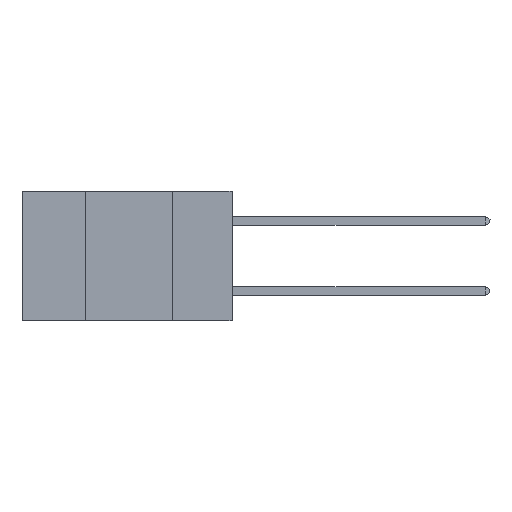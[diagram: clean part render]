
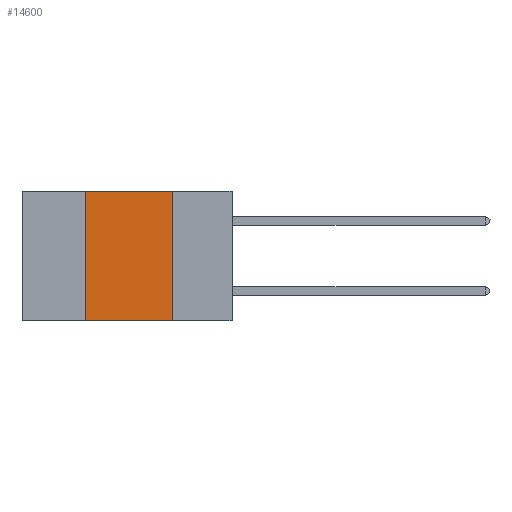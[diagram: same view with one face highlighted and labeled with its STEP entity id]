
A CAD part, left-side view. The second image highlights one B-rep face of the part: STEP entity #14600.
In plain terms, the highlighted planar face has unit normal (-1, 0, 0).
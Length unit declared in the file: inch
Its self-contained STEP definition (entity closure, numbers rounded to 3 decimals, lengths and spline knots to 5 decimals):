
#266 = DIRECTION ( 'NONE',  ( 0., -1., 0. ) ) ;
#727 = DIRECTION ( 'NONE',  ( 0., 0., -1. ) ) ;
#1215 = CARTESIAN_POINT ( 'NONE',  ( 0., 0.17, 0. ) ) ;
#2251 = VECTOR ( 'NONE', #266, 39.37008 ) ;
#2693 = CARTESIAN_POINT ( 'NONE',  ( 0., 0.6, 0. ) ) ;
#4339 = CARTESIAN_POINT ( 'NONE',  ( 0., 0.42, 0. ) ) ;
#4403 = VECTOR ( 'NONE', #10729, 39.37008 ) ;
#4668 = LINE ( 'NONE', #23076, #2251 ) ;
#6224 = CARTESIAN_POINT ( 'NONE',  ( 0., 0.6, -0.37 ) ) ;
#6250 = CARTESIAN_POINT ( 'NONE',  ( 0., 0.42, -0.37 ) ) ;
#8404 = DIRECTION ( 'NONE',  ( 1., 0., 0. ) ) ;
#8484 = VECTOR ( 'NONE', #22388, 39.37008 ) ;
#9470 = VECTOR ( 'NONE', #19108, 39.37008 ) ;
#10675 = CARTESIAN_POINT ( 'NONE',  ( 0., 0.17, 0. ) ) ;
#10729 = DIRECTION ( 'NONE',  ( 0., 0., -1. ) ) ;
#10884 = EDGE_LOOP ( 'NONE', ( #11351, #22325, #14289, #11941 ) ) ;
#11351 = ORIENTED_EDGE ( 'NONE', *, *, #20361, .F. ) ;
#11361 = LINE ( 'NONE', #18141, #8484 ) ;
#11571 = VERTEX_POINT ( 'NONE', #4339 ) ;
#11721 = LINE ( 'NONE', #1215, #4403 ) ;
#11941 = ORIENTED_EDGE ( 'NONE', *, *, #18050, .T. ) ;
#12480 = EDGE_CURVE ( 'NONE', #11571, #13008, #4668, .T. ) ;
#12697 = CARTESIAN_POINT ( 'NONE',  ( 0., 0.17, -0.37 ) ) ;
#12824 = EDGE_CURVE ( 'NONE', #21925, #11571, #11361, .T. ) ;
#13008 = VERTEX_POINT ( 'NONE', #10675 ) ;
#14289 = ORIENTED_EDGE ( 'NONE', *, *, #12824, .F. ) ;
#14600 = ADVANCED_FACE ( 'NONE', ( #19871 ), #19644, .F. ) ;
#16844 = LINE ( 'NONE', #6224, #9470 ) ;
#18050 = EDGE_CURVE ( 'NONE', #21925, #24168, #16844, .T. ) ;
#18141 = CARTESIAN_POINT ( 'NONE',  ( 0., 0.42, 0. ) ) ;
#19108 = DIRECTION ( 'NONE',  ( 0., -1., 0. ) ) ;
#19644 = PLANE ( 'NONE',  #20961 ) ;
#19871 = FACE_OUTER_BOUND ( 'NONE', #10884, .T. ) ;
#20361 = EDGE_CURVE ( 'NONE', #13008, #24168, #11721, .T. ) ;
#20961 = AXIS2_PLACEMENT_3D ( 'NONE', #2693, #8404, #727 ) ;
#21925 = VERTEX_POINT ( 'NONE', #6250 ) ;
#22325 = ORIENTED_EDGE ( 'NONE', *, *, #12480, .F. ) ;
#22388 = DIRECTION ( 'NONE',  ( 0., 0., 1. ) ) ;
#23076 = CARTESIAN_POINT ( 'NONE',  ( 0., 0.6, 0. ) ) ;
#24168 = VERTEX_POINT ( 'NONE', #12697 ) ;
